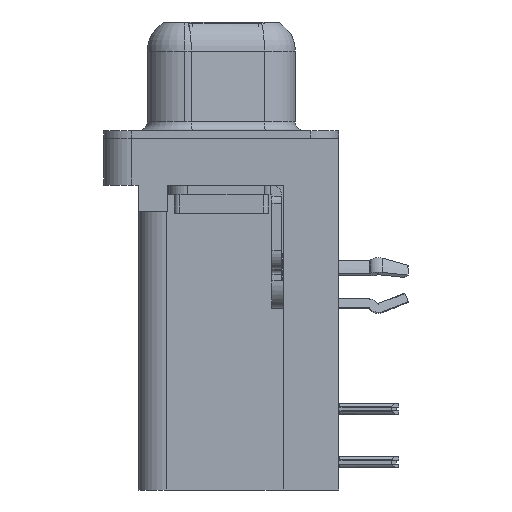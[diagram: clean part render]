
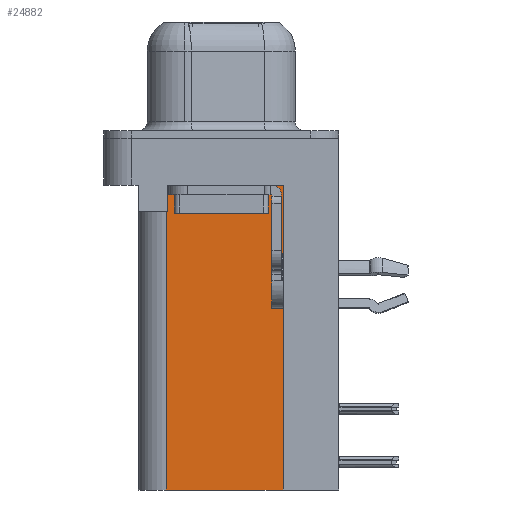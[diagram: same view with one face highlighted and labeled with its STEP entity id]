
A CAD part, left-side view. The second image highlights one B-rep face of the part: STEP entity #24882.
In plain terms, the highlighted planar face has unit normal (-1, 0, 0).
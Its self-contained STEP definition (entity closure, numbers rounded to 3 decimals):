
#3564 = EDGE_CURVE ( 'NONE', #18764, #13931, #16551, .T. ) ;
#4030 = EDGE_CURVE ( 'NONE', #18764, #7021, #8173, .T. ) ;
#5206 = DIRECTION ( 'NONE',  ( 0., 0., -1. ) ) ;
#5493 = ORIENTED_EDGE ( 'NONE', *, *, #14433, .T. ) ;
#6701 = EDGE_LOOP ( 'NONE', ( #16141, #5493, #27710, #27749, #13208, #19153 ) ) ;
#7021 = VERTEX_POINT ( 'NONE', #8237 ) ;
#7947 = CARTESIAN_POINT ( 'NONE',  ( 3.79, -3.295, -18.76 ) ) ;
#8082 = CARTESIAN_POINT ( 'NONE',  ( 3.79, 0., -3.9 ) ) ;
#8130 = CARTESIAN_POINT ( 'NONE',  ( 3.79, 2.895, -3.9 ) ) ;
#8159 = CARTESIAN_POINT ( 'NONE',  ( 3.79, 2.925, -18.76 ) ) ;
#8173 = LINE ( 'NONE', #7947, #8253 ) ;
#8237 = CARTESIAN_POINT ( 'NONE',  ( 3.79, -3.295, -2.5 ) ) ;
#8253 = VECTOR ( 'NONE', #25459, 1000. ) ;
#8534 = CARTESIAN_POINT ( 'NONE',  ( 3.79, -3.295, -18.76 ) ) ;
#10062 = VERTEX_POINT ( 'NONE', #10206 ) ;
#10206 = CARTESIAN_POINT ( 'NONE',  ( 3.79, 2.925, -3.9 ) ) ;
#10270 = EDGE_CURVE ( 'NONE', #7021, #12270, #12252, .T. ) ;
#11092 = DIRECTION ( 'NONE',  ( 0., 1., 0. ) ) ;
#11536 = DIRECTION ( 'NONE',  ( 1., 0., 0. ) ) ;
#12169 = VECTOR ( 'NONE', #37177, 1000. ) ;
#12252 = LINE ( 'NONE', #17039, #12169 ) ;
#12270 = VERTEX_POINT ( 'NONE', #22376 ) ;
#13208 = ORIENTED_EDGE ( 'NONE', *, *, #3564, .F. ) ;
#13931 = VERTEX_POINT ( 'NONE', #8159 ) ;
#14094 = FACE_OUTER_BOUND ( 'NONE', #6701, .T. ) ;
#14433 = EDGE_CURVE ( 'NONE', #12270, #17195, #32693, .T. ) ;
#15327 = LINE ( 'NONE', #8082, #29883 ) ;
#15711 = DIRECTION ( 'NONE',  ( 0., 0., 1. ) ) ;
#16054 = VECTOR ( 'NONE', #29072, 1000. ) ;
#16141 = ORIENTED_EDGE ( 'NONE', *, *, #10270, .T. ) ;
#16551 = LINE ( 'NONE', #32390, #16054 ) ;
#17039 = CARTESIAN_POINT ( 'NONE',  ( 3.79, -3.295, -2.5 ) ) ;
#17195 = VERTEX_POINT ( 'NONE', #19066 ) ;
#17251 = VECTOR ( 'NONE', #5206, 1000. ) ;
#18764 = VERTEX_POINT ( 'NONE', #25105 ) ;
#19066 = CARTESIAN_POINT ( 'NONE',  ( 3.79, 2.895, -3.9 ) ) ;
#19067 = EDGE_CURVE ( 'NONE', #13931, #10062, #23253, .T. ) ;
#19153 = ORIENTED_EDGE ( 'NONE', *, *, #4030, .T. ) ;
#22354 = VECTOR ( 'NONE', #15711, 1000. ) ;
#22376 = CARTESIAN_POINT ( 'NONE',  ( 3.79, 2.895, -2.5 ) ) ;
#23253 = LINE ( 'NONE', #33110, #22354 ) ;
#24882 = ADVANCED_FACE ( 'NONE', ( #14094 ), #26022, .F. ) ;
#25105 = CARTESIAN_POINT ( 'NONE',  ( 3.79, -3.295, -18.76 ) ) ;
#25459 = DIRECTION ( 'NONE',  ( 0., 0., 1. ) ) ;
#26022 = PLANE ( 'NONE',  #29171 ) ;
#27710 = ORIENTED_EDGE ( 'NONE', *, *, #31937, .T. ) ;
#27749 = ORIENTED_EDGE ( 'NONE', *, *, #19067, .F. ) ;
#29072 = DIRECTION ( 'NONE',  ( 0., 1., 0. ) ) ;
#29171 = AXIS2_PLACEMENT_3D ( 'NONE', #8534, #11536, #31924 ) ;
#29883 = VECTOR ( 'NONE', #11092, 1000. ) ;
#31924 = DIRECTION ( 'NONE',  ( 0., 1., 0. ) ) ;
#31937 = EDGE_CURVE ( 'NONE', #17195, #10062, #15327, .T. ) ;
#32390 = CARTESIAN_POINT ( 'NONE',  ( 3.79, -3.295, -18.76 ) ) ;
#32693 = LINE ( 'NONE', #8130, #17251 ) ;
#33110 = CARTESIAN_POINT ( 'NONE',  ( 3.79, 2.925, -18.76 ) ) ;
#37177 = DIRECTION ( 'NONE',  ( 0., 1., 0. ) ) ;
